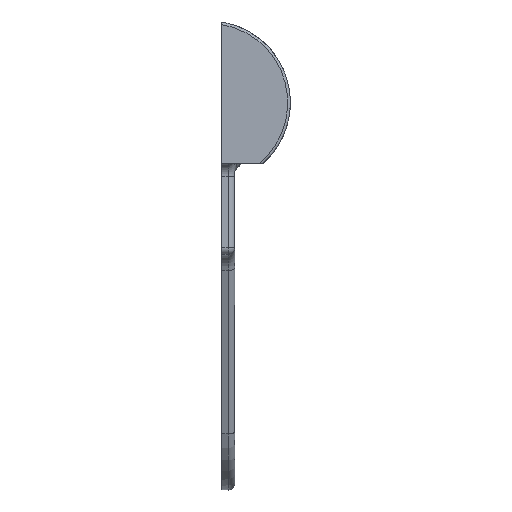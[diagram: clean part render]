
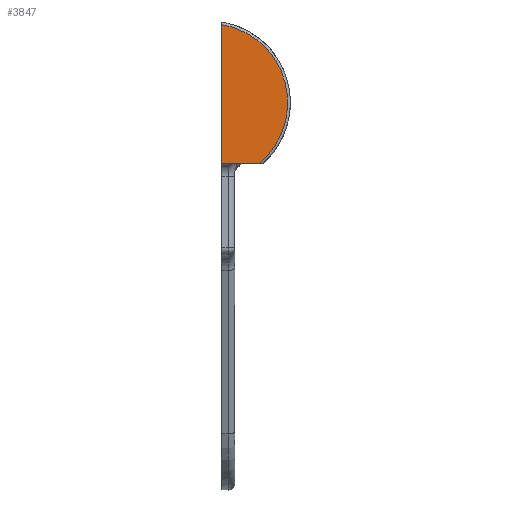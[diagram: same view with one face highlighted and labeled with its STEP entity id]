
A CAD part, top view. The second image highlights one B-rep face of the part: STEP entity #3847.
In plain terms, the highlighted planar face has unit normal (0, 0, 1).
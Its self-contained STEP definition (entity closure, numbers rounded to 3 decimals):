
#92 = AXIS2_PLACEMENT_3D ( 'NONE', #1636, #2575, #638 ) ;
#353 = VECTOR ( 'NONE', #2790, 1000. ) ;
#529 = DIRECTION ( 'NONE',  ( -1., 0., 0. ) ) ;
#638 = DIRECTION ( 'NONE',  ( 0., 1., 0. ) ) ;
#641 = CARTESIAN_POINT ( 'NONE',  ( 19.402, -20., 35. ) ) ;
#1023 = VERTEX_POINT ( 'NONE', #1765 ) ;
#1178 = ORIENTED_EDGE ( 'NONE', *, *, #3728, .F. ) ;
#1284 = LINE ( 'NONE', #4028, #353 ) ;
#1396 = LINE ( 'NONE', #3724, #2117 ) ;
#1413 = AXIS2_PLACEMENT_3D ( 'NONE', #3428, #1575, #3746 ) ;
#1575 = DIRECTION ( 'NONE',  ( 0., 0., -1. ) ) ;
#1636 = CARTESIAN_POINT ( 'NONE',  ( 5., 0., 35. ) ) ;
#1765 = CARTESIAN_POINT ( 'NONE',  ( 5., -20., 35. ) ) ;
#1797 = CARTESIAN_POINT ( 'NONE',  ( 5., 33.621, 35. ) ) ;
#2117 = VECTOR ( 'NONE', #529, 1000. ) ;
#2265 = PLANE ( 'NONE',  #92 ) ;
#2267 = FACE_OUTER_BOUND ( 'NONE', #3631, .T. ) ;
#2575 = DIRECTION ( 'NONE',  ( 0., 0., -1. ) ) ;
#2746 = VERTEX_POINT ( 'NONE', #1797 ) ;
#2790 = DIRECTION ( 'NONE',  ( 0., -1., 0. ) ) ;
#3278 = ORIENTED_EDGE ( 'NONE', *, *, #3720, .T. ) ;
#3428 = CARTESIAN_POINT ( 'NONE',  ( 0., 3.534, 35. ) ) ;
#3631 = EDGE_LOOP ( 'NONE', ( #3278, #1178, #3778 ) ) ;
#3683 = CIRCLE ( 'NONE', #1413, 30.5 ) ;
#3720 = EDGE_CURVE ( 'NONE', #2746, #1023, #1284, .T. ) ;
#3724 = CARTESIAN_POINT ( 'NONE',  ( 5., -20., 35. ) ) ;
#3728 = EDGE_CURVE ( 'NONE', #4098, #1023, #1396, .T. ) ;
#3746 = DIRECTION ( 'NONE',  ( 0., 1., 0. ) ) ;
#3748 = EDGE_CURVE ( 'NONE', #2746, #4098, #3683, .T. ) ;
#3778 = ORIENTED_EDGE ( 'NONE', *, *, #3748, .F. ) ;
#3847 = ADVANCED_FACE ( 'NONE', ( #2267 ), #2265, .F. ) ;
#4028 = CARTESIAN_POINT ( 'NONE',  ( 5., -145.897, 35. ) ) ;
#4098 = VERTEX_POINT ( 'NONE', #641 ) ;
